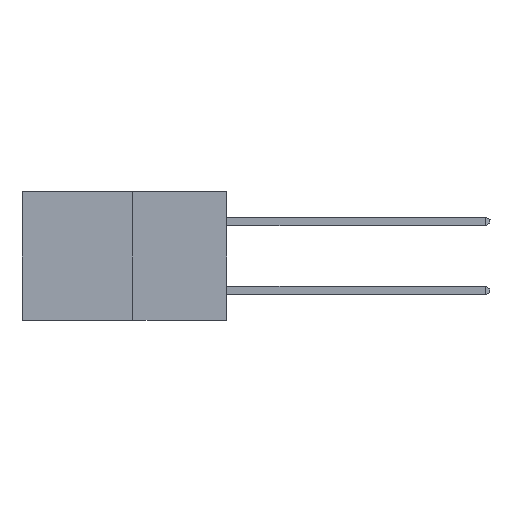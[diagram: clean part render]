
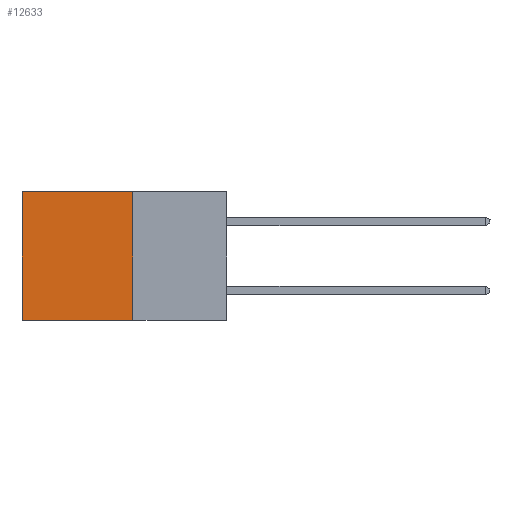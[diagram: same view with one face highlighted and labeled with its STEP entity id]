
A CAD part, left-side view. The second image highlights one B-rep face of the part: STEP entity #12633.
In plain terms, the highlighted planar face has unit normal (-1, 0, 0).
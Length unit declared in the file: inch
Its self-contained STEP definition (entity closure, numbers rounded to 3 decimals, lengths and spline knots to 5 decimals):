
#65 = CARTESIAN_POINT ( 'NONE',  ( 0.277, 0.27, -0.37 ) ) ;
#115 = DIRECTION ( 'NONE',  ( 0., 1., 0. ) ) ;
#146 = CARTESIAN_POINT ( 'NONE',  ( 0.277, 0.27, -0.37 ) ) ;
#1027 = EDGE_CURVE ( 'NONE', #29794, #24833, #12113, .T. ) ;
#1964 = CARTESIAN_POINT ( 'NONE',  ( 0.277, 0.27, -0.37 ) ) ;
#2294 = VERTEX_POINT ( 'NONE', #24386 ) ;
#2494 = DIRECTION ( 'NONE',  ( 1., 0., 0. ) ) ;
#4483 = VECTOR ( 'NONE', #30014, 39.37008 ) ;
#5249 = DIRECTION ( 'NONE',  ( 0., 1., 0. ) ) ;
#5978 = EDGE_CURVE ( 'NONE', #2294, #24833, #12662, .T. ) ;
#6445 = VECTOR ( 'NONE', #115, 39.37008 ) ;
#7055 = LINE ( 'NONE', #10114, #13465 ) ;
#7773 = VERTEX_POINT ( 'NONE', #12983 ) ;
#10114 = CARTESIAN_POINT ( 'NONE',  ( 0.277, 0.27, 0. ) ) ;
#10799 = ORIENTED_EDGE ( 'NONE', *, *, #19039, .F. ) ;
#11199 = CARTESIAN_POINT ( 'NONE',  ( 0.277, 0.27, -0.37 ) ) ;
#11915 = VECTOR ( 'NONE', #27845, 39.37008 ) ;
#12113 = LINE ( 'NONE', #146, #6445 ) ;
#12633 = ADVANCED_FACE ( 'NONE', ( #16843 ), #16782, .F. ) ;
#12662 = LINE ( 'NONE', #28046, #11915 ) ;
#12983 = CARTESIAN_POINT ( 'NONE',  ( 0.277, 0.27, 0. ) ) ;
#13465 = VECTOR ( 'NONE', #5249, 39.37008 ) ;
#14521 = ORIENTED_EDGE ( 'NONE', *, *, #5978, .T. ) ;
#16521 = CARTESIAN_POINT ( 'NONE',  ( 0.277, 0.59, -0.37 ) ) ;
#16782 = PLANE ( 'NONE',  #29353 ) ;
#16843 = FACE_OUTER_BOUND ( 'NONE', #26057, .T. ) ;
#17560 = ORIENTED_EDGE ( 'NONE', *, *, #25019, .T. ) ;
#19039 = EDGE_CURVE ( 'NONE', #7773, #29794, #28000, .T. ) ;
#19127 = DIRECTION ( 'NONE',  ( 0., 0., -1. ) ) ;
#24386 = CARTESIAN_POINT ( 'NONE',  ( 0.277, 0.59, 0. ) ) ;
#24833 = VERTEX_POINT ( 'NONE', #16521 ) ;
#25019 = EDGE_CURVE ( 'NONE', #7773, #2294, #7055, .T. ) ;
#26057 = EDGE_LOOP ( 'NONE', ( #14521, #30044, #10799, #17560 ) ) ;
#27845 = DIRECTION ( 'NONE',  ( 0., 0., -1. ) ) ;
#28000 = LINE ( 'NONE', #1964, #4483 ) ;
#28046 = CARTESIAN_POINT ( 'NONE',  ( 0.277, 0.59, -0.37 ) ) ;
#29353 = AXIS2_PLACEMENT_3D ( 'NONE', #65, #2494, #19127 ) ;
#29794 = VERTEX_POINT ( 'NONE', #11199 ) ;
#30014 = DIRECTION ( 'NONE',  ( 0., 0., -1. ) ) ;
#30044 = ORIENTED_EDGE ( 'NONE', *, *, #1027, .F. ) ;
